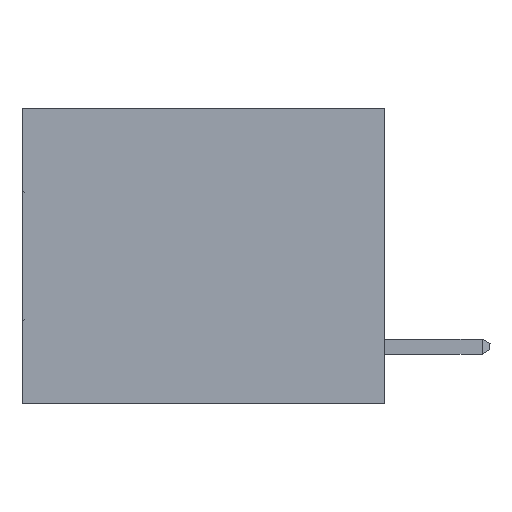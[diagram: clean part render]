
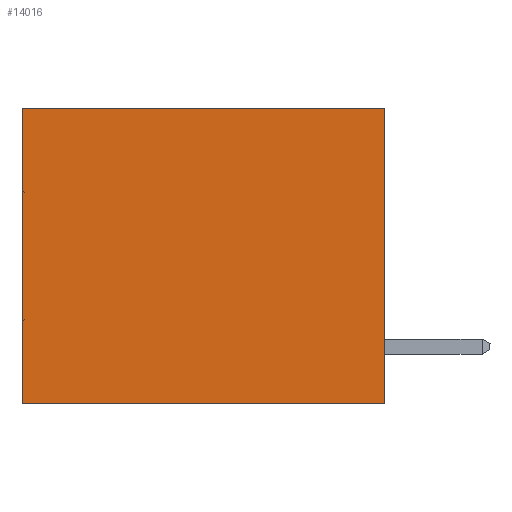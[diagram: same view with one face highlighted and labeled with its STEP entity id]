
A CAD part, left-side view. The second image highlights one B-rep face of the part: STEP entity #14016.
In plain terms, the highlighted planar face has unit normal (-1, 0, 0).
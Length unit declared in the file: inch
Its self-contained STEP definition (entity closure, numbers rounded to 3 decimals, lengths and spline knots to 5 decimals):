
#247 = PLANE ( 'NONE',  #10540 ) ;
#1878 = VERTEX_POINT ( 'NONE', #3309 ) ;
#1992 = EDGE_CURVE ( 'NONE', #2519, #1878, #26174, .T. ) ;
#2208 = ORIENTED_EDGE ( 'NONE', *, *, #26818, .T. ) ;
#2519 = VERTEX_POINT ( 'NONE', #29265 ) ;
#2738 = CARTESIAN_POINT ( 'NONE',  ( 0.3165, 0., -0.49 ) ) ;
#3309 = CARTESIAN_POINT ( 'NONE',  ( 0.3165, 0.6, -0.49 ) ) ;
#3550 = CARTESIAN_POINT ( 'NONE',  ( 0.3165, 0.6, -0.49 ) ) ;
#5196 = ORIENTED_EDGE ( 'NONE', *, *, #23613, .F. ) ;
#8569 = DIRECTION ( 'NONE',  ( 0., 0., -1. ) ) ;
#8641 = EDGE_CURVE ( 'NONE', #11124, #1878, #27082, .T. ) ;
#8901 = FACE_OUTER_BOUND ( 'NONE', #29070, .T. ) ;
#9020 = ORIENTED_EDGE ( 'NONE', *, *, #8641, .F. ) ;
#9617 = CARTESIAN_POINT ( 'NONE',  ( 0.3165, 0., 0. ) ) ;
#10540 = AXIS2_PLACEMENT_3D ( 'NONE', #19135, #16325, #8569 ) ;
#11124 = VERTEX_POINT ( 'NONE', #13719 ) ;
#11524 = VECTOR ( 'NONE', #18949, 39.37008 ) ;
#12604 = CARTESIAN_POINT ( 'NONE',  ( 0.3165, 0., 0. ) ) ;
#13006 = VECTOR ( 'NONE', #19931, 39.37008 ) ;
#13719 = CARTESIAN_POINT ( 'NONE',  ( 0.3165, 0., -0.49 ) ) ;
#14016 = ADVANCED_FACE ( 'NONE', ( #8901 ), #247, .F. ) ;
#14468 = DIRECTION ( 'NONE',  ( 0., 0., -1. ) ) ;
#16325 = DIRECTION ( 'NONE',  ( 1., 0., 0. ) ) ;
#17076 = ORIENTED_EDGE ( 'NONE', *, *, #1992, .T. ) ;
#18949 = DIRECTION ( 'NONE',  ( 0., 0., -1. ) ) ;
#19135 = CARTESIAN_POINT ( 'NONE',  ( 0.3165, 0., -0.49 ) ) ;
#19931 = DIRECTION ( 'NONE',  ( 0., 1., 0. ) ) ;
#20013 = VECTOR ( 'NONE', #31799, 39.37008 ) ;
#22839 = CARTESIAN_POINT ( 'NONE',  ( 0.3165, 0., -0.49 ) ) ;
#23613 = EDGE_CURVE ( 'NONE', #32457, #11124, #34250, .T. ) ;
#25778 = VECTOR ( 'NONE', #14468, 39.37008 ) ;
#26174 = LINE ( 'NONE', #3550, #25778 ) ;
#26818 = EDGE_CURVE ( 'NONE', #32457, #2519, #28470, .T. ) ;
#27082 = LINE ( 'NONE', #2738, #20013 ) ;
#28470 = LINE ( 'NONE', #12604, #13006 ) ;
#29070 = EDGE_LOOP ( 'NONE', ( #17076, #9020, #5196, #2208 ) ) ;
#29265 = CARTESIAN_POINT ( 'NONE',  ( 0.3165, 0.6, 0. ) ) ;
#31799 = DIRECTION ( 'NONE',  ( 0., 1., 0. ) ) ;
#32457 = VERTEX_POINT ( 'NONE', #9617 ) ;
#34250 = LINE ( 'NONE', #22839, #11524 ) ;
